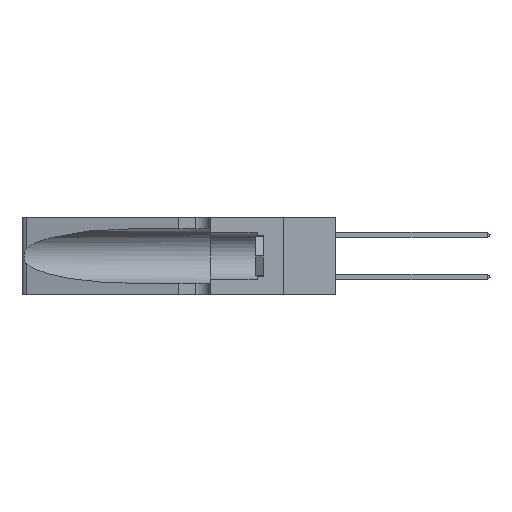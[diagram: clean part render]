
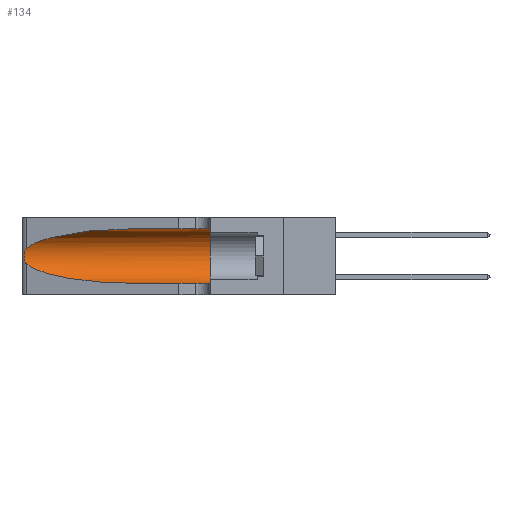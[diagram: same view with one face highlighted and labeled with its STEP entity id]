
A CAD part, left-side view. The second image highlights one B-rep face of the part: STEP entity #134.
In plain terms, the highlighted cylindrical face has radius 3.308 mm (diameter 6.617 mm), a partial arc.
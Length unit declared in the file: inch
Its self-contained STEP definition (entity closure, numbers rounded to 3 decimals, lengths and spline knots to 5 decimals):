
#61 = ORIENTED_EDGE ( 'NONE', *, *, #10076, .T. ) ;
#134 = ADVANCED_FACE ( 'NONE', ( #9626 ), #35809, .F. ) ;
#447 = DIRECTION ( 'NONE',  ( 0., 1., 0. ) ) ;
#1213 = CIRCLE ( 'NONE', #21717, 0.13025 ) ;
#1721 = EDGE_CURVE ( 'NONE', #22592, #43918, #32924, .T. ) ;
#2385 = AXIS2_PLACEMENT_3D ( 'NONE', #4979, #12480, #16249 ) ;
#3027 = CARTESIAN_POINT ( 'NONE',  ( 0.25789, 1.23486, 0.15765 ) ) ;
#3647 = CARTESIAN_POINT ( 'NONE',  ( 0.1305, 1.61858, 0.05475 ) ) ;
#4979 = CARTESIAN_POINT ( 'NONE',  ( 0.1305, 1.61858, 0.185 ) ) ;
#6636 = CARTESIAN_POINT ( 'NONE',  ( 0.25487, 1.22718, 0.22369 ) ) ;
#6795 = CARTESIAN_POINT ( 'NONE',  ( 0.25555, 1.22993, 0.14849 ) ) ;
#7331 = CARTESIAN_POINT ( 'NONE',  ( 0.25487, 1.22718, 0.22369 ) ) ;
#9626 = FACE_OUTER_BOUND ( 'NONE', #22010, .T. ) ;
#9786 = EDGE_CURVE ( 'NONE', #22592, #35968, #28759, .T. ) ;
#10076 = EDGE_CURVE ( 'NONE', #23474, #47981, #35394, .T. ) ;
#12480 = DIRECTION ( 'NONE',  ( 0., -1., 0. ) ) ;
#12493 = VERTEX_POINT ( 'NONE', #16692 ) ;
#14140 = CARTESIAN_POINT ( 'NONE',  ( 0.25787, 1.23484, 0.2124 ) ) ;
#15347 = CARTESIAN_POINT ( 'NONE',  ( 0.18966, 0.96281, 0.05475 ) ) ;
#15629 =( BOUNDED_CURVE ( )  B_SPLINE_CURVE ( 3, ( #44523, #40761, #15347, #26048 ),
 .UNSPECIFIED., .F., .F. ) 
 B_SPLINE_CURVE_WITH_KNOTS ( ( 4, 4 ),
 ( 3.44316, 4.71239 ),
 .UNSPECIFIED. ) 
 CURVE ( )  GEOMETRIC_REPRESENTATION_ITEM ( )  RATIONAL_B_SPLINE_CURVE ( ( 1., 0.87, 0.87, 1. ) ) 
 REPRESENTATION_ITEM ( '' )  );
#16043 = CARTESIAN_POINT ( 'NONE',  ( 0.1305, 0.35, 0.31525 ) ) ;
#16249 = DIRECTION ( 'NONE',  ( 0., 0., -1. ) ) ;
#16692 = CARTESIAN_POINT ( 'NONE',  ( 0.25487, 1.22718, 0.14631 ) ) ;
#17634 = B_SPLINE_CURVE_WITH_KNOTS ( 'NONE', 3,
 ( #6636, #28973, #36376, #14140, #40113, #17904, #43853, #21667, #47601, #25402, #3027, #29119, #6795, #32855 ),
 .UNSPECIFIED., .F., .F.,
 ( 4, 2, 2, 2, 2, 2, 4 ),
 ( 0., 0.00027, 0.00053, 0.00107, 0.0016, 0.00187, 0.00214 ),
 .UNSPECIFIED. ) ;
#17904 = CARTESIAN_POINT ( 'NONE',  ( 0.26018, 1.23835, 0.19895 ) ) ;
#18081 = CARTESIAN_POINT ( 'NONE',  ( 0.1305, 0.72297, 0.31525 ) ) ;
#18606 = VECTOR ( 'NONE', #42864, 39.37008 ) ;
#18759 = ORIENTED_EDGE ( 'NONE', *, *, #19249, .T. ) ;
#18770 = CARTESIAN_POINT ( 'NONE',  ( 0.1305, 0.72297, 0.05475 ) ) ;
#19249 = EDGE_CURVE ( 'NONE', #12493, #23474, #15629, .T. ) ;
#20964 = CARTESIAN_POINT ( 'NONE',  ( 0.1305, 0.72297, 0.31525 ) ) ;
#21667 = CARTESIAN_POINT ( 'NONE',  ( 0.26075, 1.23896, 0.178 ) ) ;
#21717 = AXIS2_PLACEMENT_3D ( 'NONE', #22799, #447, #26526 ) ;
#22010 = EDGE_LOOP ( 'NONE', ( #33828, #37302, #18759, #61, #41943, #33285 ) ) ;
#22592 = VERTEX_POINT ( 'NONE', #20964 ) ;
#22799 = CARTESIAN_POINT ( 'NONE',  ( 0.1305, 0.35, 0.185 ) ) ;
#22873 = CARTESIAN_POINT ( 'NONE',  ( 0.1305, 0.35, 0.05475 ) ) ;
#23474 = VERTEX_POINT ( 'NONE', #18770 ) ;
#24016 = EDGE_CURVE ( 'NONE', #43918, #12493, #17634, .T. ) ;
#25402 = CARTESIAN_POINT ( 'NONE',  ( 0.25856, 1.23593, 0.16098 ) ) ;
#25994 = DIRECTION ( 'NONE',  ( 0., -1., 0. ) ) ;
#26048 = CARTESIAN_POINT ( 'NONE',  ( 0.1305, 0.72297, 0.05475 ) ) ;
#26526 = DIRECTION ( 'NONE',  ( 0., 0., 1. ) ) ;
#28133 = CARTESIAN_POINT ( 'NONE',  ( 0.1305, 1.61858, 0.31525 ) ) ;
#28759 = LINE ( 'NONE', #28133, #18606 ) ;
#28973 = CARTESIAN_POINT ( 'NONE',  ( 0.25555, 1.22994, 0.2215 ) ) ;
#29119 = CARTESIAN_POINT ( 'NONE',  ( 0.25639, 1.23186, 0.15144 ) ) ;
#32855 = CARTESIAN_POINT ( 'NONE',  ( 0.25487, 1.22718, 0.14631 ) ) ;
#32924 =( BOUNDED_CURVE ( )  B_SPLINE_CURVE ( 3, ( #18081, #40303, #36555, #44045 ),
 .UNSPECIFIED., .F., .F. ) 
 B_SPLINE_CURVE_WITH_KNOTS ( ( 4, 4 ),
 ( 1.5708, 2.84003 ),
 .UNSPECIFIED. ) 
 CURVE ( )  GEOMETRIC_REPRESENTATION_ITEM ( )  RATIONAL_B_SPLINE_CURVE ( ( 1., 0.87, 0.87, 1. ) ) 
 REPRESENTATION_ITEM ( '' )  );
#33285 = ORIENTED_EDGE ( 'NONE', *, *, #9786, .F. ) ;
#33828 = ORIENTED_EDGE ( 'NONE', *, *, #1721, .T. ) ;
#35235 = EDGE_CURVE ( 'NONE', #35968, #47981, #1213, .T. ) ;
#35394 = LINE ( 'NONE', #3647, #46443 ) ;
#35809 = CYLINDRICAL_SURFACE ( 'NONE', #2385, 0.13025 ) ;
#35968 = VERTEX_POINT ( 'NONE', #16043 ) ;
#36376 = CARTESIAN_POINT ( 'NONE',  ( 0.25639, 1.23184, 0.21858 ) ) ;
#36555 = CARTESIAN_POINT ( 'NONE',  ( 0.2373, 1.15595, 0.28018 ) ) ;
#37302 = ORIENTED_EDGE ( 'NONE', *, *, #24016, .T. ) ;
#40113 = CARTESIAN_POINT ( 'NONE',  ( 0.25854, 1.2359, 0.20912 ) ) ;
#40303 = CARTESIAN_POINT ( 'NONE',  ( 0.18966, 0.96281, 0.31525 ) ) ;
#40761 = CARTESIAN_POINT ( 'NONE',  ( 0.2373, 1.15595, 0.08982 ) ) ;
#41943 = ORIENTED_EDGE ( 'NONE', *, *, #35235, .F. ) ;
#42864 = DIRECTION ( 'NONE',  ( 0., -1., 0. ) ) ;
#43853 = CARTESIAN_POINT ( 'NONE',  ( 0.26075, 1.23896, 0.19203 ) ) ;
#43918 = VERTEX_POINT ( 'NONE', #7331 ) ;
#44045 = CARTESIAN_POINT ( 'NONE',  ( 0.25487, 1.22718, 0.22369 ) ) ;
#44523 = CARTESIAN_POINT ( 'NONE',  ( 0.25487, 1.22718, 0.14631 ) ) ;
#46443 = VECTOR ( 'NONE', #25994, 39.37008 ) ;
#47601 = CARTESIAN_POINT ( 'NONE',  ( 0.26017, 1.23833, 0.17102 ) ) ;
#47981 = VERTEX_POINT ( 'NONE', #22873 ) ;
